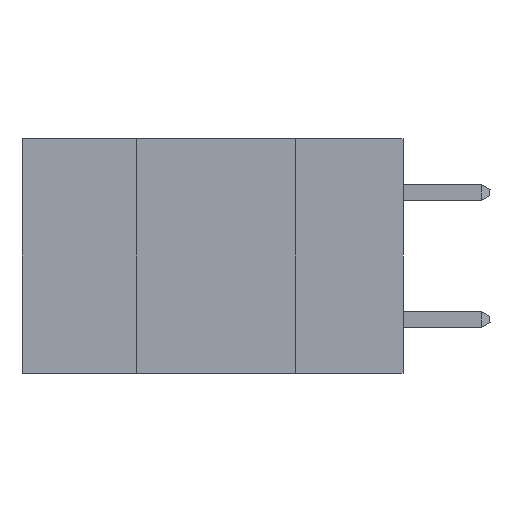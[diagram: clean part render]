
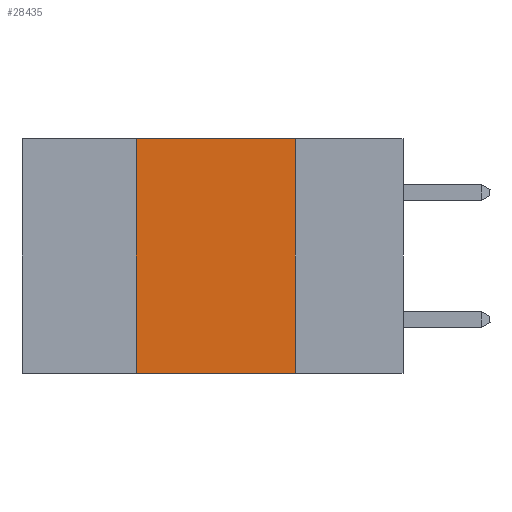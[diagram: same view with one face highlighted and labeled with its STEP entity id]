
A CAD part, left-side view. The second image highlights one B-rep face of the part: STEP entity #28435.
In plain terms, the highlighted planar face has unit normal (-1, 0, 0).
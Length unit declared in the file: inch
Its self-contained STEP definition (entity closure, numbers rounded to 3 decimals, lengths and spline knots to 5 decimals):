
#129 = FACE_OUTER_BOUND ( 'NONE', #12993, .T. ) ;
#755 = VECTOR ( 'NONE', #33879, 39.37008 ) ;
#2105 = ORIENTED_EDGE ( 'NONE', *, *, #10431, .F. ) ;
#2162 = CARTESIAN_POINT ( 'NONE',  ( 0., 0.6, 0. ) ) ;
#2802 = DIRECTION ( 'NONE',  ( 0., -1., 0. ) ) ;
#2931 = VERTEX_POINT ( 'NONE', #20096 ) ;
#4817 = LINE ( 'NONE', #2162, #35373 ) ;
#5540 = EDGE_CURVE ( 'NONE', #13492, #23690, #4817, .T. ) ;
#5790 = CARTESIAN_POINT ( 'NONE',  ( 0., 0.17, 0. ) ) ;
#7122 = VECTOR ( 'NONE', #13969, 39.37008 ) ;
#10431 = EDGE_CURVE ( 'NONE', #23690, #2931, #16851, .T. ) ;
#12895 = ORIENTED_EDGE ( 'NONE', *, *, #5540, .F. ) ;
#12993 = EDGE_LOOP ( 'NONE', ( #2105, #12895, #32797, #15877 ) ) ;
#13492 = VERTEX_POINT ( 'NONE', #17277 ) ;
#13628 = VECTOR ( 'NONE', #34918, 39.37008 ) ;
#13909 = CARTESIAN_POINT ( 'NONE',  ( 0., 0.42, -0.37 ) ) ;
#13969 = DIRECTION ( 'NONE',  ( 0., -1., 0. ) ) ;
#14715 = DIRECTION ( 'NONE',  ( 0., 0., -1. ) ) ;
#14882 = EDGE_CURVE ( 'NONE', #18104, #2931, #28451, .T. ) ;
#15877 = ORIENTED_EDGE ( 'NONE', *, *, #14882, .T. ) ;
#16851 = LINE ( 'NONE', #29243, #13628 ) ;
#17277 = CARTESIAN_POINT ( 'NONE',  ( 0., 0.42, 0. ) ) ;
#18013 = CARTESIAN_POINT ( 'NONE',  ( 0., 0.6, -0.37 ) ) ;
#18104 = VERTEX_POINT ( 'NONE', #13909 ) ;
#20096 = CARTESIAN_POINT ( 'NONE',  ( 0., 0.17, -0.37 ) ) ;
#20695 = CARTESIAN_POINT ( 'NONE',  ( 0., 0.6, 0. ) ) ;
#20791 = AXIS2_PLACEMENT_3D ( 'NONE', #20695, #21095, #14715 ) ;
#21095 = DIRECTION ( 'NONE',  ( 1., 0., 0. ) ) ;
#23690 = VERTEX_POINT ( 'NONE', #5790 ) ;
#24633 = CARTESIAN_POINT ( 'NONE',  ( 0., 0.42, 0. ) ) ;
#26592 = EDGE_CURVE ( 'NONE', #18104, #13492, #31831, .T. ) ;
#26749 = PLANE ( 'NONE',  #20791 ) ;
#28435 = ADVANCED_FACE ( 'NONE', ( #129 ), #26749, .F. ) ;
#28451 = LINE ( 'NONE', #18013, #7122 ) ;
#29243 = CARTESIAN_POINT ( 'NONE',  ( 0., 0.17, 0. ) ) ;
#31831 = LINE ( 'NONE', #24633, #755 ) ;
#32797 = ORIENTED_EDGE ( 'NONE', *, *, #26592, .F. ) ;
#33879 = DIRECTION ( 'NONE',  ( 0., 0., 1. ) ) ;
#34918 = DIRECTION ( 'NONE',  ( 0., 0., -1. ) ) ;
#35373 = VECTOR ( 'NONE', #2802, 39.37008 ) ;
